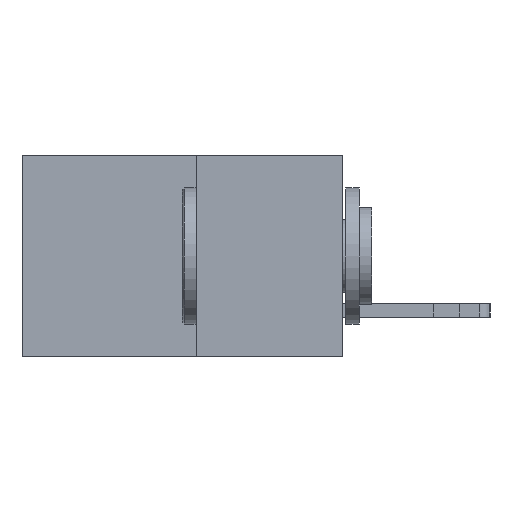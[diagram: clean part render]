
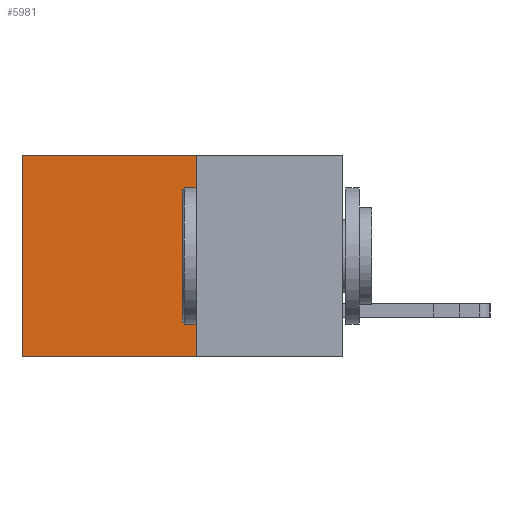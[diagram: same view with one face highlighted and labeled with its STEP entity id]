
A CAD part, left-side view. The second image highlights one B-rep face of the part: STEP entity #5981.
In plain terms, the highlighted planar face has unit normal (-1, 0, 0).
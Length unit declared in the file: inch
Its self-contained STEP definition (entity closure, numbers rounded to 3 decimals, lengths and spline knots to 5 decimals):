
#292 = VERTEX_POINT ( 'NONE', #5075 ) ;
#2628 = VECTOR ( 'NONE', #9807, 39.37008 ) ;
#2871 = DIRECTION ( 'NONE',  ( 0., 0., -1. ) ) ;
#3403 = VERTEX_POINT ( 'NONE', #22476 ) ;
#4133 = LINE ( 'NONE', #9897, #25515 ) ;
#4867 = EDGE_CURVE ( 'NONE', #14043, #3403, #18893, .T. ) ;
#4965 = ORIENTED_EDGE ( 'NONE', *, *, #19663, .T. ) ;
#5075 = CARTESIAN_POINT ( 'NONE',  ( 0.277, 0.59, -0.37 ) ) ;
#5092 = LINE ( 'NONE', #18178, #16443 ) ;
#5267 = ORIENTED_EDGE ( 'NONE', *, *, #9480, .T. ) ;
#5448 = VERTEX_POINT ( 'NONE', #22737 ) ;
#5981 = ADVANCED_FACE ( 'NONE', ( #7874 ), #12279, .F. ) ;
#6283 = DIRECTION ( 'NONE',  ( 1., 0., 0. ) ) ;
#7102 = AXIS2_PLACEMENT_3D ( 'NONE', #10261, #6283, #20352 ) ;
#7874 = FACE_OUTER_BOUND ( 'NONE', #24582, .T. ) ;
#8152 = LINE ( 'NONE', #21830, #2628 ) ;
#8202 = DIRECTION ( 'NONE',  ( 0., 1., 0. ) ) ;
#9480 = EDGE_CURVE ( 'NONE', #5448, #292, #4133, .T. ) ;
#9807 = DIRECTION ( 'NONE',  ( 0., 1., 0. ) ) ;
#9897 = CARTESIAN_POINT ( 'NONE',  ( 0.277, 0.59, -0.37 ) ) ;
#10261 = CARTESIAN_POINT ( 'NONE',  ( 0.277, 0.27, -0.37 ) ) ;
#12279 = PLANE ( 'NONE',  #7102 ) ;
#14043 = VERTEX_POINT ( 'NONE', #16616 ) ;
#16443 = VECTOR ( 'NONE', #8202, 39.37008 ) ;
#16453 = ORIENTED_EDGE ( 'NONE', *, *, #22088, .F. ) ;
#16616 = CARTESIAN_POINT ( 'NONE',  ( 0.277, 0.27, 0. ) ) ;
#18178 = CARTESIAN_POINT ( 'NONE',  ( 0.277, 0.27, -0.37 ) ) ;
#18893 = LINE ( 'NONE', #19074, #23576 ) ;
#19074 = CARTESIAN_POINT ( 'NONE',  ( 0.277, 0.27, -0.37 ) ) ;
#19663 = EDGE_CURVE ( 'NONE', #14043, #5448, #8152, .T. ) ;
#20352 = DIRECTION ( 'NONE',  ( 0., 0., -1. ) ) ;
#21830 = CARTESIAN_POINT ( 'NONE',  ( 0.277, 0.27, 0. ) ) ;
#22088 = EDGE_CURVE ( 'NONE', #3403, #292, #5092, .T. ) ;
#22476 = CARTESIAN_POINT ( 'NONE',  ( 0.277, 0.27, -0.37 ) ) ;
#22737 = CARTESIAN_POINT ( 'NONE',  ( 0.277, 0.59, 0. ) ) ;
#23576 = VECTOR ( 'NONE', #2871, 39.37008 ) ;
#23900 = DIRECTION ( 'NONE',  ( 0., 0., -1. ) ) ;
#24465 = ORIENTED_EDGE ( 'NONE', *, *, #4867, .F. ) ;
#24582 = EDGE_LOOP ( 'NONE', ( #5267, #16453, #24465, #4965 ) ) ;
#25515 = VECTOR ( 'NONE', #23900, 39.37008 ) ;
